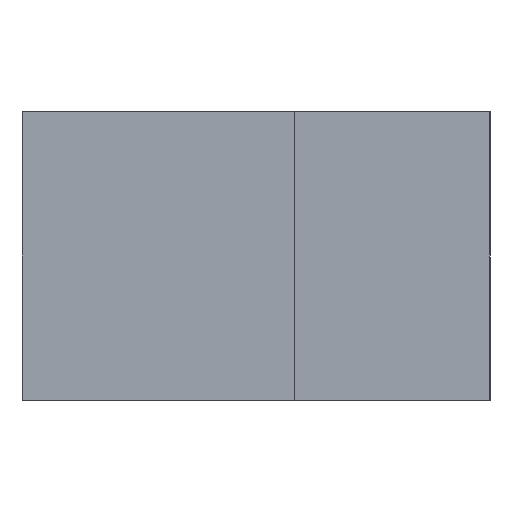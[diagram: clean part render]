
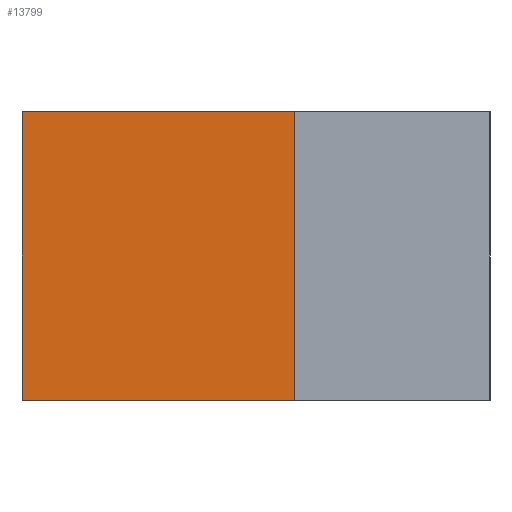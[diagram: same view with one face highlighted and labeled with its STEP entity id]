
A CAD part, left-side view. The second image highlights one B-rep face of the part: STEP entity #13799.
In plain terms, the highlighted planar face has unit normal (-1, 0, 0).
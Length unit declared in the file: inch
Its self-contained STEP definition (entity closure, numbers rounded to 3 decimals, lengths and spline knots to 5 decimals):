
#556 = DIRECTION ( 'NONE',  ( 0., 0., -1. ) ) ;
#914 = EDGE_CURVE ( 'NONE', #14801, #13809, #6139, .T. ) ;
#1058 = VERTEX_POINT ( 'NONE', #15052 ) ;
#1315 = LINE ( 'NONE', #6864, #8401 ) ;
#2382 = ORIENTED_EDGE ( 'NONE', *, *, #11390, .T. ) ;
#2649 = DIRECTION ( 'NONE',  ( 0., 1., 0. ) ) ;
#2685 = CARTESIAN_POINT ( 'NONE',  ( 0.2875, 0.25, -0.37 ) ) ;
#2842 = ORIENTED_EDGE ( 'NONE', *, *, #11017, .F. ) ;
#2987 = DIRECTION ( 'NONE',  ( 0., 0., -1. ) ) ;
#3122 = VECTOR ( 'NONE', #2649, 39.37008 ) ;
#3204 = EDGE_CURVE ( 'NONE', #14801, #9935, #1315, .T. ) ;
#3867 = VECTOR ( 'NONE', #2987, 39.37008 ) ;
#5702 = CARTESIAN_POINT ( 'NONE',  ( 0.2875, 0.25, 0. ) ) ;
#6139 = LINE ( 'NONE', #14779, #3122 ) ;
#6398 = CARTESIAN_POINT ( 'NONE',  ( 0.2875, 0.25, 0. ) ) ;
#6864 = CARTESIAN_POINT ( 'NONE',  ( 0.2875, 0.25, 0. ) ) ;
#6953 = DIRECTION ( 'NONE',  ( 0., 0., -1. ) ) ;
#7354 = ORIENTED_EDGE ( 'NONE', *, *, #3204, .F. ) ;
#7604 = AXIS2_PLACEMENT_3D ( 'NONE', #5702, #14407, #6953 ) ;
#7624 = LINE ( 'NONE', #11764, #3867 ) ;
#8315 = ORIENTED_EDGE ( 'NONE', *, *, #914, .T. ) ;
#8401 = VECTOR ( 'NONE', #556, 39.37008 ) ;
#9545 = DIRECTION ( 'NONE',  ( 0., 1., 0. ) ) ;
#9935 = VERTEX_POINT ( 'NONE', #2685 ) ;
#10637 = CARTESIAN_POINT ( 'NONE',  ( 0.2875, 0.6, 0. ) ) ;
#10780 = CARTESIAN_POINT ( 'NONE',  ( 0.2875, 0.25, -0.37 ) ) ;
#11017 = EDGE_CURVE ( 'NONE', #9935, #1058, #13510, .T. ) ;
#11390 = EDGE_CURVE ( 'NONE', #13809, #1058, #7624, .T. ) ;
#11764 = CARTESIAN_POINT ( 'NONE',  ( 0.2875, 0.6, 0. ) ) ;
#12728 = VECTOR ( 'NONE', #9545, 39.37008 ) ;
#13170 = PLANE ( 'NONE',  #7604 ) ;
#13510 = LINE ( 'NONE', #10780, #12728 ) ;
#13606 = FACE_OUTER_BOUND ( 'NONE', #14195, .T. ) ;
#13799 = ADVANCED_FACE ( 'NONE', ( #13606 ), #13170, .F. ) ;
#13809 = VERTEX_POINT ( 'NONE', #10637 ) ;
#14195 = EDGE_LOOP ( 'NONE', ( #2382, #2842, #7354, #8315 ) ) ;
#14407 = DIRECTION ( 'NONE',  ( 1., 0., 0. ) ) ;
#14779 = CARTESIAN_POINT ( 'NONE',  ( 0.2875, 0.25, 0. ) ) ;
#14801 = VERTEX_POINT ( 'NONE', #6398 ) ;
#15052 = CARTESIAN_POINT ( 'NONE',  ( 0.2875, 0.6, -0.37 ) ) ;
